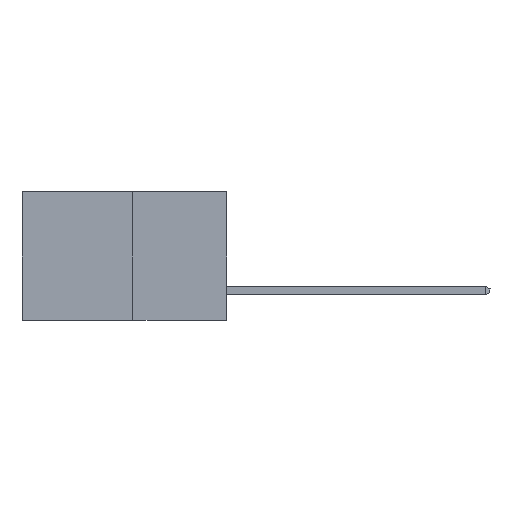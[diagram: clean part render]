
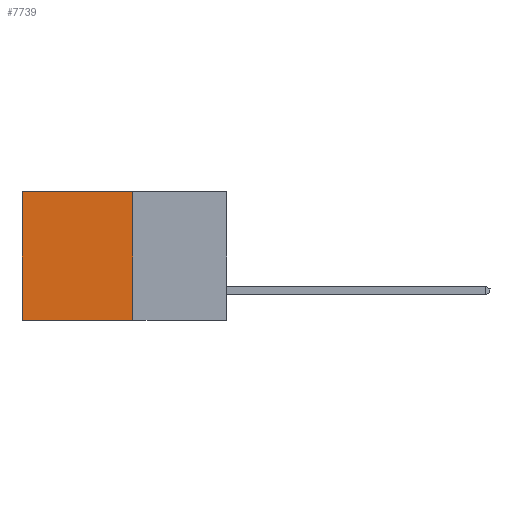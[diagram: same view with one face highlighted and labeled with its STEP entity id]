
A CAD part, left-side view. The second image highlights one B-rep face of the part: STEP entity #7739.
In plain terms, the highlighted planar face has unit normal (-1, 0, 0).
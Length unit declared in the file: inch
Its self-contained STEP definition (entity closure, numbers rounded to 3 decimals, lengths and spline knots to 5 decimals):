
#311 = DIRECTION ( 'NONE',  ( 0., 1., 0. ) ) ;
#799 = DIRECTION ( 'NONE',  ( 0., 0., -1. ) ) ;
#1394 = CARTESIAN_POINT ( 'NONE',  ( 0.277, 0.27, 0. ) ) ;
#1420 = CARTESIAN_POINT ( 'NONE',  ( 0.277, 0.27, -0.37 ) ) ;
#1740 = EDGE_CURVE ( 'NONE', #16179, #3016, #16858, .T. ) ;
#1949 = CARTESIAN_POINT ( 'NONE',  ( 0.277, 0.27, -0.37 ) ) ;
#2385 = EDGE_CURVE ( 'NONE', #15563, #15901, #12996, .T. ) ;
#2913 = CARTESIAN_POINT ( 'NONE',  ( 0.277, 0.59, 0. ) ) ;
#3016 = VERTEX_POINT ( 'NONE', #11059 ) ;
#3393 = DIRECTION ( 'NONE',  ( 0., 0., -1. ) ) ;
#3513 = DIRECTION ( 'NONE',  ( 0., 1., 0. ) ) ;
#3643 = CARTESIAN_POINT ( 'NONE',  ( 0.277, 0.27, -0.37 ) ) ;
#4188 = EDGE_CURVE ( 'NONE', #3016, #15901, #5021, .T. ) ;
#4557 = ORIENTED_EDGE ( 'NONE', *, *, #2385, .T. ) ;
#5011 = ORIENTED_EDGE ( 'NONE', *, *, #4188, .F. ) ;
#5021 = LINE ( 'NONE', #3643, #12373 ) ;
#6260 = PLANE ( 'NONE',  #17838 ) ;
#7160 = EDGE_CURVE ( 'NONE', #16179, #15563, #10484, .T. ) ;
#7739 = ADVANCED_FACE ( 'NONE', ( #8154 ), #6260, .F. ) ;
#7979 = CARTESIAN_POINT ( 'NONE',  ( 0.277, 0.59, -0.37 ) ) ;
#8154 = FACE_OUTER_BOUND ( 'NONE', #15339, .T. ) ;
#8964 = ORIENTED_EDGE ( 'NONE', *, *, #1740, .F. ) ;
#9412 = VECTOR ( 'NONE', #11432, 39.37008 ) ;
#10016 = VECTOR ( 'NONE', #311, 39.37008 ) ;
#10484 = LINE ( 'NONE', #13431, #10016 ) ;
#11059 = CARTESIAN_POINT ( 'NONE',  ( 0.277, 0.27, -0.37 ) ) ;
#11432 = DIRECTION ( 'NONE',  ( 0., 0., -1. ) ) ;
#11847 = CARTESIAN_POINT ( 'NONE',  ( 0.277, 0.59, -0.37 ) ) ;
#12172 = DIRECTION ( 'NONE',  ( 1., 0., 0. ) ) ;
#12373 = VECTOR ( 'NONE', #3513, 39.37008 ) ;
#12996 = LINE ( 'NONE', #11847, #16864 ) ;
#13279 = ORIENTED_EDGE ( 'NONE', *, *, #7160, .T. ) ;
#13431 = CARTESIAN_POINT ( 'NONE',  ( 0.277, 0.27, 0. ) ) ;
#15339 = EDGE_LOOP ( 'NONE', ( #4557, #5011, #8964, #13279 ) ) ;
#15563 = VERTEX_POINT ( 'NONE', #2913 ) ;
#15901 = VERTEX_POINT ( 'NONE', #7979 ) ;
#16179 = VERTEX_POINT ( 'NONE', #1394 ) ;
#16858 = LINE ( 'NONE', #1420, #9412 ) ;
#16864 = VECTOR ( 'NONE', #799, 39.37008 ) ;
#17838 = AXIS2_PLACEMENT_3D ( 'NONE', #1949, #12172, #3393 ) ;
